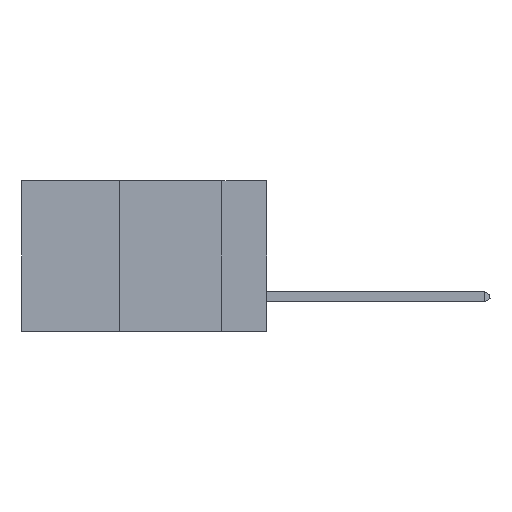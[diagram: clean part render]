
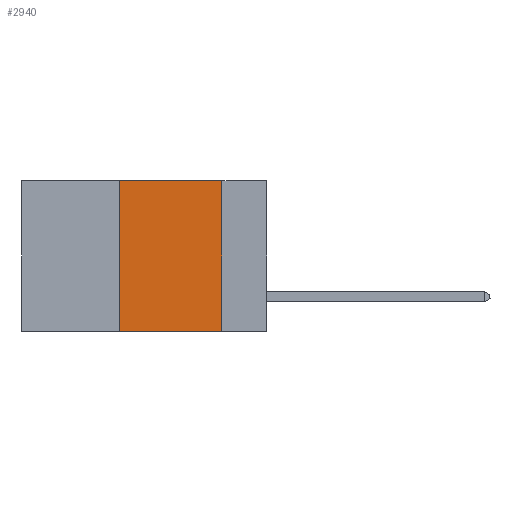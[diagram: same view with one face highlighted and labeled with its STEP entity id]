
A CAD part, left-side view. The second image highlights one B-rep face of the part: STEP entity #2940.
In plain terms, the highlighted planar face has unit normal (-1, 0, 0).
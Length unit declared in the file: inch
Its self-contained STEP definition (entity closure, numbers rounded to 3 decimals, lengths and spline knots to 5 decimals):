
#250 = VERTEX_POINT ( 'NONE', #10608 ) ;
#363 = EDGE_CURVE ( 'NONE', #13660, #250, #3727, .T. ) ;
#702 = VECTOR ( 'NONE', #751, 39.37008 ) ;
#751 = DIRECTION ( 'NONE',  ( 0., -1., 0. ) ) ;
#1020 = FACE_OUTER_BOUND ( 'NONE', #14190, .T. ) ;
#1570 = VECTOR ( 'NONE', #4499, 39.37008 ) ;
#2018 = VERTEX_POINT ( 'NONE', #17549 ) ;
#2940 = ADVANCED_FACE ( 'NONE', ( #1020 ), #9935, .F. ) ;
#3727 = LINE ( 'NONE', #4594, #10715 ) ;
#3856 = ORIENTED_EDGE ( 'NONE', *, *, #363, .F. ) ;
#4133 = ORIENTED_EDGE ( 'NONE', *, *, #5235, .F. ) ;
#4196 = DIRECTION ( 'NONE',  ( 0., -1., 0. ) ) ;
#4499 = DIRECTION ( 'NONE',  ( 0., 0., -1. ) ) ;
#4594 = CARTESIAN_POINT ( 'NONE',  ( 0., 0.36, 0. ) ) ;
#4613 = LINE ( 'NONE', #10213, #18155 ) ;
#5175 = DIRECTION ( 'NONE',  ( 1., 0., 0. ) ) ;
#5235 = EDGE_CURVE ( 'NONE', #250, #8401, #19021, .T. ) ;
#5307 = CARTESIAN_POINT ( 'NONE',  ( 0., 0.6, 0. ) ) ;
#7159 = ORIENTED_EDGE ( 'NONE', *, *, #9141, .T. ) ;
#7706 = DIRECTION ( 'NONE',  ( 0., 0., 1. ) ) ;
#7900 = EDGE_CURVE ( 'NONE', #8401, #2018, #15530, .T. ) ;
#8085 = CARTESIAN_POINT ( 'NONE',  ( 0., 0.36, -0.37 ) ) ;
#8401 = VERTEX_POINT ( 'NONE', #10693 ) ;
#9141 = EDGE_CURVE ( 'NONE', #13660, #2018, #4613, .T. ) ;
#9935 = PLANE ( 'NONE',  #19943 ) ;
#10213 = CARTESIAN_POINT ( 'NONE',  ( 0., 0.6, -0.37 ) ) ;
#10587 = CARTESIAN_POINT ( 'NONE',  ( 0., 0.11, 0. ) ) ;
#10608 = CARTESIAN_POINT ( 'NONE',  ( 0., 0.36, 0. ) ) ;
#10693 = CARTESIAN_POINT ( 'NONE',  ( 0., 0.11, 0. ) ) ;
#10715 = VECTOR ( 'NONE', #7706, 39.37008 ) ;
#11623 = ORIENTED_EDGE ( 'NONE', *, *, #7900, .F. ) ;
#13197 = CARTESIAN_POINT ( 'NONE',  ( 0., 0.6, 0. ) ) ;
#13660 = VERTEX_POINT ( 'NONE', #8085 ) ;
#14190 = EDGE_LOOP ( 'NONE', ( #11623, #4133, #3856, #7159 ) ) ;
#15530 = LINE ( 'NONE', #10587, #1570 ) ;
#17549 = CARTESIAN_POINT ( 'NONE',  ( 0., 0.11, -0.37 ) ) ;
#17887 = DIRECTION ( 'NONE',  ( 0., 0., -1. ) ) ;
#18155 = VECTOR ( 'NONE', #4196, 39.37008 ) ;
#19021 = LINE ( 'NONE', #13197, #702 ) ;
#19943 = AXIS2_PLACEMENT_3D ( 'NONE', #5307, #5175, #17887 ) ;
